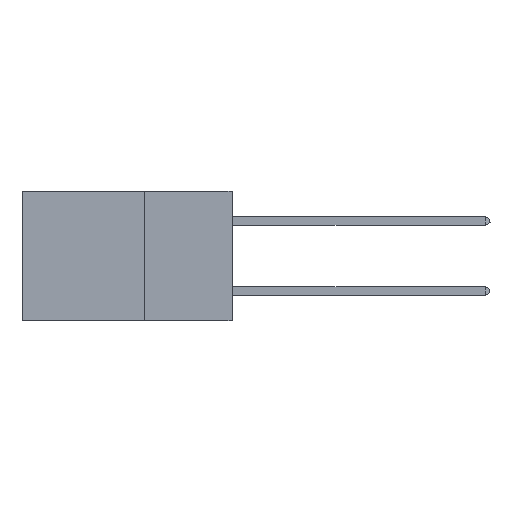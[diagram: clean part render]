
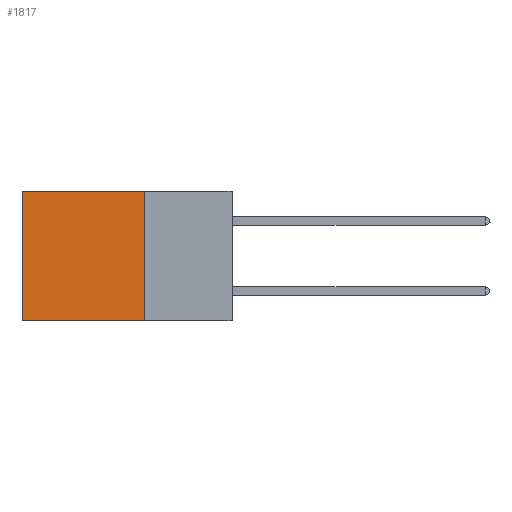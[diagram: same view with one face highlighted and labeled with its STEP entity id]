
A CAD part, left-side view. The second image highlights one B-rep face of the part: STEP entity #1817.
In plain terms, the highlighted planar face has unit normal (-1, 0, 0).
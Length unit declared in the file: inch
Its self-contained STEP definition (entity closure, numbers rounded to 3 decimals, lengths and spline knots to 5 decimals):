
#188 = PLANE ( 'NONE',  #15081 ) ;
#893 = DIRECTION ( 'NONE',  ( 0., 0., -1. ) ) ;
#1817 = ADVANCED_FACE ( 'NONE', ( #24172 ), #188, .F. ) ;
#2569 = EDGE_CURVE ( 'NONE', #11707, #7170, #3939, .T. ) ;
#3429 = CARTESIAN_POINT ( 'NONE',  ( 0.2875, 0.25, 0. ) ) ;
#3494 = CARTESIAN_POINT ( 'NONE',  ( 0.2875, 0.25, 0. ) ) ;
#3515 = VERTEX_POINT ( 'NONE', #3494 ) ;
#3939 = LINE ( 'NONE', #14618, #11031 ) ;
#4055 = LINE ( 'NONE', #18882, #22956 ) ;
#5266 = CARTESIAN_POINT ( 'NONE',  ( 0.2875, 0.25, 0. ) ) ;
#5475 = LINE ( 'NONE', #3429, #6069 ) ;
#6069 = VECTOR ( 'NONE', #9117, 39.37008 ) ;
#6986 = CARTESIAN_POINT ( 'NONE',  ( 0.2875, 0.25, -0.37 ) ) ;
#7170 = VERTEX_POINT ( 'NONE', #21251 ) ;
#7984 = ORIENTED_EDGE ( 'NONE', *, *, #9093, .T. ) ;
#8971 = VERTEX_POINT ( 'NONE', #6986 ) ;
#9093 = EDGE_CURVE ( 'NONE', #3515, #11707, #11621, .T. ) ;
#9117 = DIRECTION ( 'NONE',  ( 0., 0., -1. ) ) ;
#9430 = VECTOR ( 'NONE', #15569, 39.37008 ) ;
#11031 = VECTOR ( 'NONE', #893, 39.37008 ) ;
#11621 = LINE ( 'NONE', #5266, #9430 ) ;
#11707 = VERTEX_POINT ( 'NONE', #22892 ) ;
#12995 = DIRECTION ( 'NONE',  ( 0., 1., 0. ) ) ;
#14317 = ORIENTED_EDGE ( 'NONE', *, *, #2569, .T. ) ;
#14397 = ORIENTED_EDGE ( 'NONE', *, *, #24843, .F. ) ;
#14618 = CARTESIAN_POINT ( 'NONE',  ( 0.2875, 0.6, 0. ) ) ;
#15081 = AXIS2_PLACEMENT_3D ( 'NONE', #25185, #15262, #20210 ) ;
#15262 = DIRECTION ( 'NONE',  ( 1., 0., 0. ) ) ;
#15569 = DIRECTION ( 'NONE',  ( 0., 1., 0. ) ) ;
#15992 = ORIENTED_EDGE ( 'NONE', *, *, #16195, .F. ) ;
#16195 = EDGE_CURVE ( 'NONE', #8971, #7170, #4055, .T. ) ;
#18882 = CARTESIAN_POINT ( 'NONE',  ( 0.2875, 0.25, -0.37 ) ) ;
#20210 = DIRECTION ( 'NONE',  ( 0., 0., -1. ) ) ;
#21251 = CARTESIAN_POINT ( 'NONE',  ( 0.2875, 0.6, -0.37 ) ) ;
#22892 = CARTESIAN_POINT ( 'NONE',  ( 0.2875, 0.6, 0. ) ) ;
#22956 = VECTOR ( 'NONE', #12995, 39.37008 ) ;
#23528 = EDGE_LOOP ( 'NONE', ( #14317, #15992, #14397, #7984 ) ) ;
#24172 = FACE_OUTER_BOUND ( 'NONE', #23528, .T. ) ;
#24843 = EDGE_CURVE ( 'NONE', #3515, #8971, #5475, .T. ) ;
#25185 = CARTESIAN_POINT ( 'NONE',  ( 0.2875, 0.25, 0. ) ) ;
